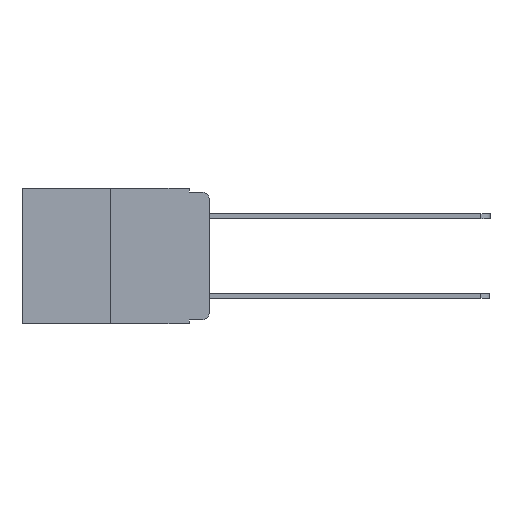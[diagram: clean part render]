
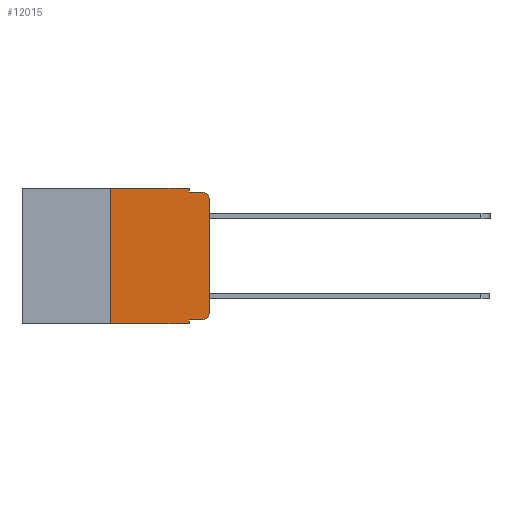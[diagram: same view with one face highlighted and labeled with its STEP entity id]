
A CAD part, left-side view. The second image highlights one B-rep face of the part: STEP entity #12015.
In plain terms, the highlighted planar face has unit normal (-1, 0, 0).
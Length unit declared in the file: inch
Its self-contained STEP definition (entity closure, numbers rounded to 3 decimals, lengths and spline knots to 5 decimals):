
#91 = EDGE_CURVE ( 'NONE', #6852, #2622, #1294, .T. ) ;
#113 = DIRECTION ( 'NONE',  ( 0., 0., -1. ) ) ;
#165 = CARTESIAN_POINT ( 'NONE',  ( 0., 0.25, -0.343 ) ) ;
#206 = VECTOR ( 'NONE', #19077, 39.37008 ) ;
#390 = DIRECTION ( 'NONE',  ( 0., -1., 0. ) ) ;
#1207 = VERTEX_POINT ( 'NONE', #14758 ) ;
#1294 = LINE ( 'NONE', #13247, #9599 ) ;
#1379 = DIRECTION ( 'NONE',  ( -1., 0., 0. ) ) ;
#1383 = VERTEX_POINT ( 'NONE', #10142 ) ;
#2622 = VERTEX_POINT ( 'NONE', #9589 ) ;
#2764 = ORIENTED_EDGE ( 'NONE', *, *, #3088, .T. ) ;
#2773 = CARTESIAN_POINT ( 'NONE',  ( 0., 0., 0. ) ) ;
#2922 = CARTESIAN_POINT ( 'NONE',  ( 0., 0.051, -0.343 ) ) ;
#3088 = EDGE_CURVE ( 'NONE', #5144, #12711, #7460, .T. ) ;
#4425 = DIRECTION ( 'NONE',  ( 0., 0., 1. ) ) ;
#4479 = VERTEX_POINT ( 'NONE', #13224 ) ;
#4803 = CARTESIAN_POINT ( 'NONE',  ( 0., 0.473, 0. ) ) ;
#5144 = VERTEX_POINT ( 'NONE', #19472 ) ;
#5210 = LINE ( 'NONE', #8366, #206 ) ;
#5542 = ORIENTED_EDGE ( 'NONE', *, *, #91, .F. ) ;
#5807 = EDGE_CURVE ( 'NONE', #6852, #19717, #7794, .T. ) ;
#6004 = VECTOR ( 'NONE', #20046, 39.37008 ) ;
#6214 = LINE ( 'NONE', #16670, #14207 ) ;
#6533 = EDGE_LOOP ( 'NONE', ( #20041, #8675, #15422, #9953, #7572, #5542, #16639, #7106, #2764, #14075 ) ) ;
#6830 = EDGE_CURVE ( 'NONE', #1383, #1207, #6214, .T. ) ;
#6852 = VERTEX_POINT ( 'NONE', #165 ) ;
#7100 = CARTESIAN_POINT ( 'NONE',  ( 0., 0.051, -0.333 ) ) ;
#7106 = ORIENTED_EDGE ( 'NONE', *, *, #13691, .F. ) ;
#7271 = VECTOR ( 'NONE', #14074, 39.37008 ) ;
#7460 = LINE ( 'NONE', #7100, #15347 ) ;
#7519 = EDGE_CURVE ( 'NONE', #16878, #17025, #9058, .T. ) ;
#7542 = CARTESIAN_POINT ( 'NONE',  ( 0., 0.02, -0.01 ) ) ;
#7572 = ORIENTED_EDGE ( 'NONE', *, *, #8156, .F. ) ;
#7592 = AXIS2_PLACEMENT_3D ( 'NONE', #8652, #19317, #10282 ) ;
#7794 = LINE ( 'NONE', #17959, #7271 ) ;
#8156 = EDGE_CURVE ( 'NONE', #2622, #1383, #16953, .T. ) ;
#8366 = CARTESIAN_POINT ( 'NONE',  ( 0., 0.051, -0.01 ) ) ;
#8652 = CARTESIAN_POINT ( 'NONE',  ( 0., 0.02, -0.313 ) ) ;
#8675 = ORIENTED_EDGE ( 'NONE', *, *, #7519, .T. ) ;
#8876 = CARTESIAN_POINT ( 'NONE',  ( 0., 0., -0.03 ) ) ;
#9058 = CIRCLE ( 'NONE', #11903, 0.02 ) ;
#9472 = CARTESIAN_POINT ( 'NONE',  ( 0., 0.051, 0. ) ) ;
#9589 = CARTESIAN_POINT ( 'NONE',  ( 0., 0.25, 0. ) ) ;
#9599 = VECTOR ( 'NONE', #13955, 39.37008 ) ;
#9953 = ORIENTED_EDGE ( 'NONE', *, *, #6830, .F. ) ;
#10098 = DIRECTION ( 'NONE',  ( 1., 0., 0. ) ) ;
#10134 = DIRECTION ( 'NONE',  ( 0., 0., -1. ) ) ;
#10142 = CARTESIAN_POINT ( 'NONE',  ( 0., 0.051, 0. ) ) ;
#10282 = DIRECTION ( 'NONE',  ( 0., 0., -1. ) ) ;
#10803 = LINE ( 'NONE', #2773, #11304 ) ;
#11304 = VECTOR ( 'NONE', #4425, 39.37008 ) ;
#11368 = LINE ( 'NONE', #9472, #6004 ) ;
#11903 = AXIS2_PLACEMENT_3D ( 'NONE', #15823, #1379, #12819 ) ;
#12015 = ADVANCED_FACE ( 'NONE', ( #19798 ), #13189, .F. ) ;
#12620 = EDGE_CURVE ( 'NONE', #12711, #4479, #16840, .T. ) ;
#12711 = VERTEX_POINT ( 'NONE', #16557 ) ;
#12819 = DIRECTION ( 'NONE',  ( 0., 0., -1. ) ) ;
#13002 = VECTOR ( 'NONE', #20318, 39.37008 ) ;
#13189 = PLANE ( 'NONE',  #13768 ) ;
#13224 = CARTESIAN_POINT ( 'NONE',  ( 0., 0., -0.313 ) ) ;
#13247 = CARTESIAN_POINT ( 'NONE',  ( 0., 0.25, 0. ) ) ;
#13691 = EDGE_CURVE ( 'NONE', #5144, #19717, #11368, .T. ) ;
#13768 = AXIS2_PLACEMENT_3D ( 'NONE', #19138, #10098, #113 ) ;
#13948 = EDGE_CURVE ( 'NONE', #1207, #17025, #5210, .T. ) ;
#13955 = DIRECTION ( 'NONE',  ( 0., 0., 1. ) ) ;
#14074 = DIRECTION ( 'NONE',  ( 0., -1., 0. ) ) ;
#14075 = ORIENTED_EDGE ( 'NONE', *, *, #12620, .T. ) ;
#14207 = VECTOR ( 'NONE', #10134, 39.37008 ) ;
#14758 = CARTESIAN_POINT ( 'NONE',  ( 0., 0.051, -0.01 ) ) ;
#15347 = VECTOR ( 'NONE', #390, 39.37008 ) ;
#15422 = ORIENTED_EDGE ( 'NONE', *, *, #13948, .F. ) ;
#15823 = CARTESIAN_POINT ( 'NONE',  ( 0., 0.02, -0.03 ) ) ;
#16557 = CARTESIAN_POINT ( 'NONE',  ( 0., 0.02, -0.333 ) ) ;
#16639 = ORIENTED_EDGE ( 'NONE', *, *, #5807, .T. ) ;
#16670 = CARTESIAN_POINT ( 'NONE',  ( 0., 0.051, 0. ) ) ;
#16840 = CIRCLE ( 'NONE', #7592, 0.02 ) ;
#16878 = VERTEX_POINT ( 'NONE', #8876 ) ;
#16953 = LINE ( 'NONE', #4803, #13002 ) ;
#17025 = VERTEX_POINT ( 'NONE', #7542 ) ;
#17959 = CARTESIAN_POINT ( 'NONE',  ( 0., 0.473, -0.343 ) ) ;
#19077 = DIRECTION ( 'NONE',  ( 0., -1., 0. ) ) ;
#19138 = CARTESIAN_POINT ( 'NONE',  ( 0., 0.473, 0. ) ) ;
#19317 = DIRECTION ( 'NONE',  ( -1., 0., 0. ) ) ;
#19472 = CARTESIAN_POINT ( 'NONE',  ( 0., 0.051, -0.333 ) ) ;
#19669 = EDGE_CURVE ( 'NONE', #4479, #16878, #10803, .T. ) ;
#19717 = VERTEX_POINT ( 'NONE', #2922 ) ;
#19798 = FACE_OUTER_BOUND ( 'NONE', #6533, .T. ) ;
#20041 = ORIENTED_EDGE ( 'NONE', *, *, #19669, .T. ) ;
#20046 = DIRECTION ( 'NONE',  ( 0., 0., -1. ) ) ;
#20318 = DIRECTION ( 'NONE',  ( 0., -1., 0. ) ) ;
